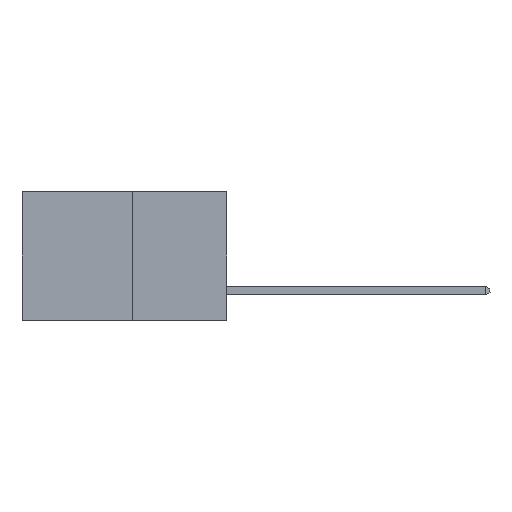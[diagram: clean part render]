
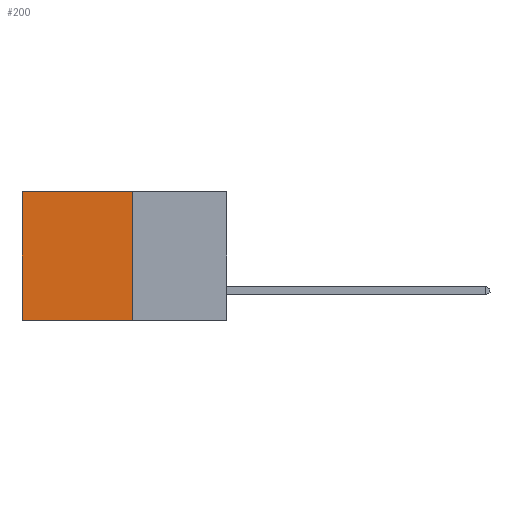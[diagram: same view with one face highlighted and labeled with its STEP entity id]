
A CAD part, left-side view. The second image highlights one B-rep face of the part: STEP entity #200.
In plain terms, the highlighted planar face has unit normal (-1, 0, 0).
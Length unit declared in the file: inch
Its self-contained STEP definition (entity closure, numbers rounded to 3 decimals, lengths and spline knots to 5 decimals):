
#200 = ADVANCED_FACE ( 'NONE', ( #4030 ), #2865, .F. ) ;
#826 = ORIENTED_EDGE ( 'NONE', *, *, #7123, .F. ) ;
#906 = CARTESIAN_POINT ( 'NONE',  ( 0.277, 0.59, 0. ) ) ;
#1784 = VERTEX_POINT ( 'NONE', #906 ) ;
#2036 = DIRECTION ( 'NONE',  ( 0., 0., -1. ) ) ;
#2116 = CARTESIAN_POINT ( 'NONE',  ( 0.277, 0.27, -0.37 ) ) ;
#2163 = DIRECTION ( 'NONE',  ( 0., 1., 0. ) ) ;
#2865 = PLANE ( 'NONE',  #3435 ) ;
#3224 = ORIENTED_EDGE ( 'NONE', *, *, #7103, .T. ) ;
#3321 = VECTOR ( 'NONE', #2163, 39.37008 ) ;
#3435 = AXIS2_PLACEMENT_3D ( 'NONE', #7975, #7328, #2036 ) ;
#3511 = VERTEX_POINT ( 'NONE', #5362 ) ;
#3707 = CARTESIAN_POINT ( 'NONE',  ( 0.277, 0.59, -0.37 ) ) ;
#4030 = FACE_OUTER_BOUND ( 'NONE', #10193, .T. ) ;
#4417 = LINE ( 'NONE', #5369, #8489 ) ;
#4578 = DIRECTION ( 'NONE',  ( 0., 0., -1. ) ) ;
#5101 = EDGE_CURVE ( 'NONE', #7171, #3511, #9299, .T. ) ;
#5249 = VECTOR ( 'NONE', #6080, 39.37008 ) ;
#5362 = CARTESIAN_POINT ( 'NONE',  ( 0.277, 0.59, -0.37 ) ) ;
#5369 = CARTESIAN_POINT ( 'NONE',  ( 0.277, 0.27, -0.37 ) ) ;
#5496 = VERTEX_POINT ( 'NONE', #9862 ) ;
#6080 = DIRECTION ( 'NONE',  ( 0., 1., 0. ) ) ;
#6545 = VECTOR ( 'NONE', #6963, 39.37008 ) ;
#6810 = LINE ( 'NONE', #3707, #6545 ) ;
#6963 = DIRECTION ( 'NONE',  ( 0., 0., -1. ) ) ;
#7103 = EDGE_CURVE ( 'NONE', #1784, #3511, #6810, .T. ) ;
#7123 = EDGE_CURVE ( 'NONE', #5496, #7171, #4417, .T. ) ;
#7171 = VERTEX_POINT ( 'NONE', #2116 ) ;
#7328 = DIRECTION ( 'NONE',  ( 1., 0., 0. ) ) ;
#7384 = LINE ( 'NONE', #10357, #3321 ) ;
#7975 = CARTESIAN_POINT ( 'NONE',  ( 0.277, 0.27, -0.37 ) ) ;
#8489 = VECTOR ( 'NONE', #4578, 39.37008 ) ;
#9299 = LINE ( 'NONE', #10151, #5249 ) ;
#9862 = CARTESIAN_POINT ( 'NONE',  ( 0.277, 0.27, 0. ) ) ;
#9884 = ORIENTED_EDGE ( 'NONE', *, *, #10565, .T. ) ;
#10135 = ORIENTED_EDGE ( 'NONE', *, *, #5101, .F. ) ;
#10151 = CARTESIAN_POINT ( 'NONE',  ( 0.277, 0.27, -0.37 ) ) ;
#10193 = EDGE_LOOP ( 'NONE', ( #3224, #10135, #826, #9884 ) ) ;
#10357 = CARTESIAN_POINT ( 'NONE',  ( 0.277, 0.27, 0. ) ) ;
#10565 = EDGE_CURVE ( 'NONE', #5496, #1784, #7384, .T. ) ;
